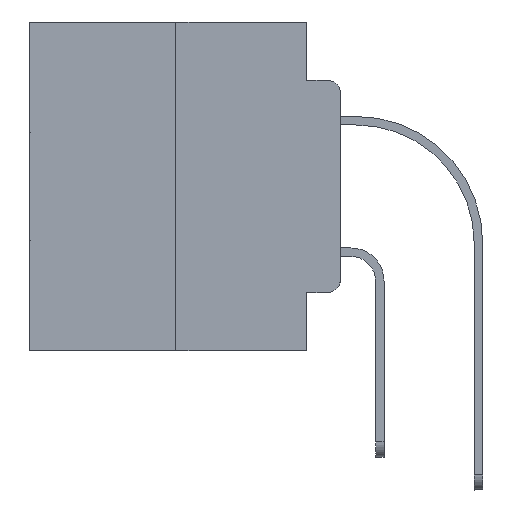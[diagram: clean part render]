
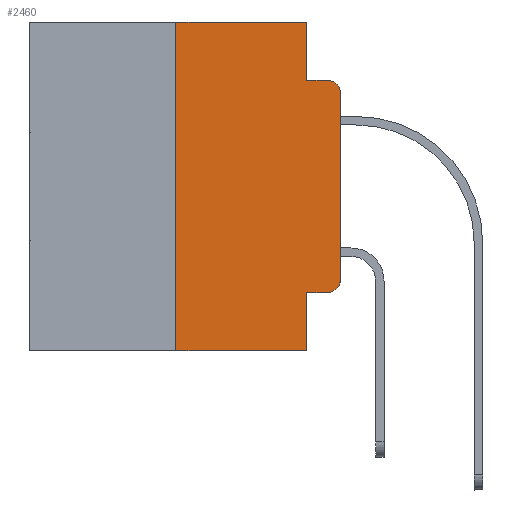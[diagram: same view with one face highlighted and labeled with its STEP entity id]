
A CAD part, left-side view. The second image highlights one B-rep face of the part: STEP entity #2460.
In plain terms, the highlighted planar face has unit normal (-1, 0, 0).
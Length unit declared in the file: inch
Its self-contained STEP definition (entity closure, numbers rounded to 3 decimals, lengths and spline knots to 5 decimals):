
#278 = CARTESIAN_POINT ( 'NONE',  ( 0., 0.02, -0.4115 ) ) ;
#1147 = DIRECTION ( 'NONE',  ( 0., -1., 0. ) ) ;
#1261 = VECTOR ( 'NONE', #15729, 39.37008 ) ;
#1670 = ORIENTED_EDGE ( 'NONE', *, *, #24406, .F. ) ;
#1709 = ORIENTED_EDGE ( 'NONE', *, *, #5220, .F. ) ;
#1860 = VERTEX_POINT ( 'NONE', #2308 ) ;
#2308 = CARTESIAN_POINT ( 'NONE',  ( 0., 0.051, -0.5 ) ) ;
#2460 = ADVANCED_FACE ( 'NONE', ( #9441 ), #9586, .F. ) ;
#2837 = CARTESIAN_POINT ( 'NONE',  ( 0., 0., -0.1085 ) ) ;
#3020 = CARTESIAN_POINT ( 'NONE',  ( 0., 0.051, 0. ) ) ;
#3747 = LINE ( 'NONE', #12414, #28295 ) ;
#3883 = DIRECTION ( 'NONE',  ( 0., -1., 0. ) ) ;
#4224 = LINE ( 'NONE', #13931, #1261 ) ;
#4757 = LINE ( 'NONE', #14019, #14130 ) ;
#5220 = EDGE_CURVE ( 'NONE', #24491, #1860, #4757, .T. ) ;
#5583 = DIRECTION ( 'NONE',  ( 0., -1., 0. ) ) ;
#6031 = CIRCLE ( 'NONE', #23237, 0.02 ) ;
#6391 = ORIENTED_EDGE ( 'NONE', *, *, #13810, .T. ) ;
#6519 = DIRECTION ( 'NONE',  ( 0., 0., -1. ) ) ;
#6719 = VECTOR ( 'NONE', #5583, 39.37008 ) ;
#6979 = LINE ( 'NONE', #23142, #9746 ) ;
#7080 = AXIS2_PLACEMENT_3D ( 'NONE', #7499, #27468, #27903 ) ;
#7181 = VECTOR ( 'NONE', #1147, 39.37008 ) ;
#7273 = DIRECTION ( 'NONE',  ( 0., -1., 0. ) ) ;
#7499 = CARTESIAN_POINT ( 'NONE',  ( 0., 0.473, 0. ) ) ;
#8089 = DIRECTION ( 'NONE',  ( 0., 0., -1. ) ) ;
#8117 = CARTESIAN_POINT ( 'NONE',  ( 0., 0.051, -0.0885 ) ) ;
#8182 = LINE ( 'NONE', #21650, #7181 ) ;
#8589 = EDGE_CURVE ( 'NONE', #28860, #26779, #27360, .T. ) ;
#8631 = ORIENTED_EDGE ( 'NONE', *, *, #8589, .F. ) ;
#9029 = VERTEX_POINT ( 'NONE', #2837 ) ;
#9232 = EDGE_CURVE ( 'NONE', #24491, #10702, #24426, .T. ) ;
#9441 = FACE_OUTER_BOUND ( 'NONE', #17627, .T. ) ;
#9586 = PLANE ( 'NONE',  #7080 ) ;
#9746 = VECTOR ( 'NONE', #7273, 39.37008 ) ;
#10173 = DIRECTION ( 'NONE',  ( -1., 0., 0. ) ) ;
#10702 = VERTEX_POINT ( 'NONE', #278 ) ;
#12407 = CARTESIAN_POINT ( 'NONE',  ( 0., 0.02, -0.1085 ) ) ;
#12414 = CARTESIAN_POINT ( 'NONE',  ( 0., 0., 0. ) ) ;
#12774 = VERTEX_POINT ( 'NONE', #3020 ) ;
#12853 = CARTESIAN_POINT ( 'NONE',  ( 0., 0.051, -0.4115 ) ) ;
#13106 = CIRCLE ( 'NONE', #26551, 0.02 ) ;
#13810 = EDGE_CURVE ( 'NONE', #28860, #1860, #8182, .T. ) ;
#13931 = CARTESIAN_POINT ( 'NONE',  ( 0., 0.051, 0. ) ) ;
#14019 = CARTESIAN_POINT ( 'NONE',  ( 0., 0.051, 0. ) ) ;
#14130 = VECTOR ( 'NONE', #27994, 39.37008 ) ;
#14973 = ORIENTED_EDGE ( 'NONE', *, *, #26795, .F. ) ;
#15623 = DIRECTION ( 'NONE',  ( 0., 0., 1. ) ) ;
#15729 = DIRECTION ( 'NONE',  ( 0., 0., -1. ) ) ;
#15797 = ORIENTED_EDGE ( 'NONE', *, *, #23786, .T. ) ;
#16935 = LINE ( 'NONE', #26123, #6719 ) ;
#17222 = ORIENTED_EDGE ( 'NONE', *, *, #22155, .F. ) ;
#17284 = CARTESIAN_POINT ( 'NONE',  ( 0., 0.02, -0.3915 ) ) ;
#17627 = EDGE_LOOP ( 'NONE', ( #28145, #25067, #14973, #1670, #17222, #8631, #6391, #1709, #19027, #15797 ) ) ;
#17795 = VERTEX_POINT ( 'NONE', #8117 ) ;
#19027 = ORIENTED_EDGE ( 'NONE', *, *, #9232, .T. ) ;
#19169 = DIRECTION ( 'NONE',  ( 0., 0., 1. ) ) ;
#19437 = CARTESIAN_POINT ( 'NONE',  ( 0., 0.25, -0.5 ) ) ;
#19986 = CARTESIAN_POINT ( 'NONE',  ( 0., 0.25, 0. ) ) ;
#21100 = CARTESIAN_POINT ( 'NONE',  ( 0., 0.02, -0.0885 ) ) ;
#21562 = CARTESIAN_POINT ( 'NONE',  ( 0., 0., -0.3915 ) ) ;
#21650 = CARTESIAN_POINT ( 'NONE',  ( 0., 0.473, -0.5 ) ) ;
#21978 = CARTESIAN_POINT ( 'NONE',  ( 0., 0.051, -0.4115 ) ) ;
#22155 = EDGE_CURVE ( 'NONE', #26779, #12774, #6979, .T. ) ;
#22793 = EDGE_CURVE ( 'NONE', #9029, #28689, #13106, .T. ) ;
#23142 = CARTESIAN_POINT ( 'NONE',  ( 0., 0.473, 0. ) ) ;
#23237 = AXIS2_PLACEMENT_3D ( 'NONE', #17284, #29311, #6519 ) ;
#23786 = EDGE_CURVE ( 'NONE', #10702, #27187, #6031, .T. ) ;
#24406 = EDGE_CURVE ( 'NONE', #12774, #17795, #4224, .T. ) ;
#24426 = LINE ( 'NONE', #12853, #25199 ) ;
#24491 = VERTEX_POINT ( 'NONE', #21978 ) ;
#25067 = ORIENTED_EDGE ( 'NONE', *, *, #22793, .T. ) ;
#25199 = VECTOR ( 'NONE', #3883, 39.37008 ) ;
#25716 = VECTOR ( 'NONE', #15623, 39.37008 ) ;
#26123 = CARTESIAN_POINT ( 'NONE',  ( 0., 0.051, -0.0885 ) ) ;
#26551 = AXIS2_PLACEMENT_3D ( 'NONE', #12407, #10173, #8089 ) ;
#26779 = VERTEX_POINT ( 'NONE', #28824 ) ;
#26795 = EDGE_CURVE ( 'NONE', #17795, #28689, #16935, .T. ) ;
#27187 = VERTEX_POINT ( 'NONE', #21562 ) ;
#27360 = LINE ( 'NONE', #19986, #25716 ) ;
#27468 = DIRECTION ( 'NONE',  ( 1., 0., 0. ) ) ;
#27903 = DIRECTION ( 'NONE',  ( 0., 0., -1. ) ) ;
#27994 = DIRECTION ( 'NONE',  ( 0., 0., -1. ) ) ;
#28145 = ORIENTED_EDGE ( 'NONE', *, *, #28435, .T. ) ;
#28295 = VECTOR ( 'NONE', #19169, 39.37008 ) ;
#28435 = EDGE_CURVE ( 'NONE', #27187, #9029, #3747, .T. ) ;
#28689 = VERTEX_POINT ( 'NONE', #21100 ) ;
#28824 = CARTESIAN_POINT ( 'NONE',  ( 0., 0.25, 0. ) ) ;
#28860 = VERTEX_POINT ( 'NONE', #19437 ) ;
#29311 = DIRECTION ( 'NONE',  ( -1., 0., 0. ) ) ;
